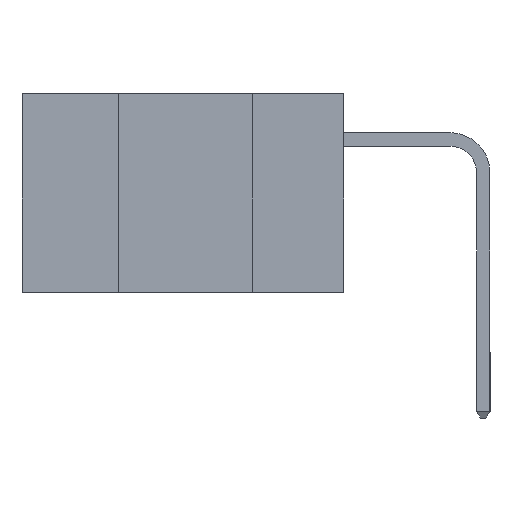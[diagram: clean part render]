
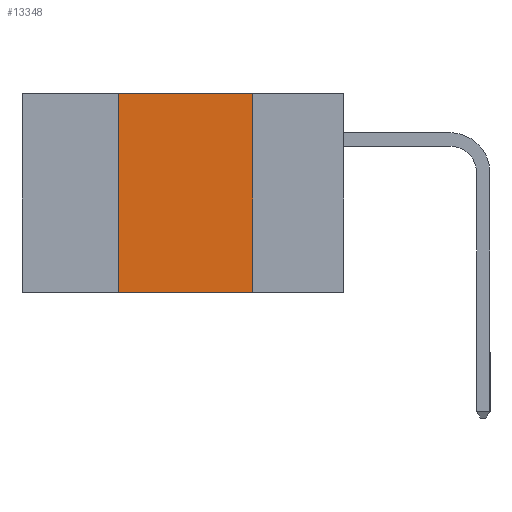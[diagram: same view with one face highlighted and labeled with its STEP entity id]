
A CAD part, left-side view. The second image highlights one B-rep face of the part: STEP entity #13348.
In plain terms, the highlighted planar face has unit normal (-1, 0, 0).
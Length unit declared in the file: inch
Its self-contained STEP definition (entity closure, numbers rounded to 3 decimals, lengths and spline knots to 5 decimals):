
#1278 = CARTESIAN_POINT ( 'NONE',  ( 0., 0.17, -0.37 ) ) ;
#1516 = EDGE_CURVE ( 'NONE', #22129, #10350, #5264, .T. ) ;
#1616 = LINE ( 'NONE', #8625, #15521 ) ;
#3662 = CARTESIAN_POINT ( 'NONE',  ( 0., 0.17, -0.37 ) ) ;
#4121 = VERTEX_POINT ( 'NONE', #10405 ) ;
#4821 = VERTEX_POINT ( 'NONE', #17992 ) ;
#5264 = LINE ( 'NONE', #3662, #8647 ) ;
#6106 = CARTESIAN_POINT ( 'NONE',  ( 0., 0.42, -0.37 ) ) ;
#6895 = DIRECTION ( 'NONE',  ( 0., -1., 0. ) ) ;
#7008 = FACE_OUTER_BOUND ( 'NONE', #8417, .T. ) ;
#8417 = EDGE_LOOP ( 'NONE', ( #11511, #9609, #10868, #9445 ) ) ;
#8625 = CARTESIAN_POINT ( 'NONE',  ( 0., 0.6, -0.37 ) ) ;
#8647 = VECTOR ( 'NONE', #21287, 39.37008 ) ;
#8896 = EDGE_CURVE ( 'NONE', #4121, #4821, #21667, .T. ) ;
#9189 = EDGE_CURVE ( 'NONE', #4121, #10350, #1616, .T. ) ;
#9445 = ORIENTED_EDGE ( 'NONE', *, *, #9189, .T. ) ;
#9609 = ORIENTED_EDGE ( 'NONE', *, *, #20780, .F. ) ;
#10072 = CARTESIAN_POINT ( 'NONE',  ( 0., 0.17, 0. ) ) ;
#10135 = CARTESIAN_POINT ( 'NONE',  ( 0., 0.6, 0. ) ) ;
#10350 = VERTEX_POINT ( 'NONE', #1278 ) ;
#10405 = CARTESIAN_POINT ( 'NONE',  ( 0., 0.42, -0.37 ) ) ;
#10868 = ORIENTED_EDGE ( 'NONE', *, *, #8896, .F. ) ;
#11066 = LINE ( 'NONE', #18107, #13827 ) ;
#11511 = ORIENTED_EDGE ( 'NONE', *, *, #1516, .F. ) ;
#12919 = DIRECTION ( 'NONE',  ( 0., 0., 1. ) ) ;
#13348 = ADVANCED_FACE ( 'NONE', ( #7008 ), #20630, .F. ) ;
#13827 = VECTOR ( 'NONE', #21546, 39.37008 ) ;
#14865 = AXIS2_PLACEMENT_3D ( 'NONE', #10135, #15569, #19362 ) ;
#15521 = VECTOR ( 'NONE', #6895, 39.37008 ) ;
#15569 = DIRECTION ( 'NONE',  ( 1., 0., 0. ) ) ;
#16987 = VECTOR ( 'NONE', #12919, 39.37008 ) ;
#17992 = CARTESIAN_POINT ( 'NONE',  ( 0., 0.42, 0. ) ) ;
#18107 = CARTESIAN_POINT ( 'NONE',  ( 0., 0.6, 0. ) ) ;
#19362 = DIRECTION ( 'NONE',  ( 0., 0., -1. ) ) ;
#20630 = PLANE ( 'NONE',  #14865 ) ;
#20780 = EDGE_CURVE ( 'NONE', #4821, #22129, #11066, .T. ) ;
#21287 = DIRECTION ( 'NONE',  ( 0., 0., -1. ) ) ;
#21546 = DIRECTION ( 'NONE',  ( 0., -1., 0. ) ) ;
#21667 = LINE ( 'NONE', #6106, #16987 ) ;
#22129 = VERTEX_POINT ( 'NONE', #10072 ) ;
